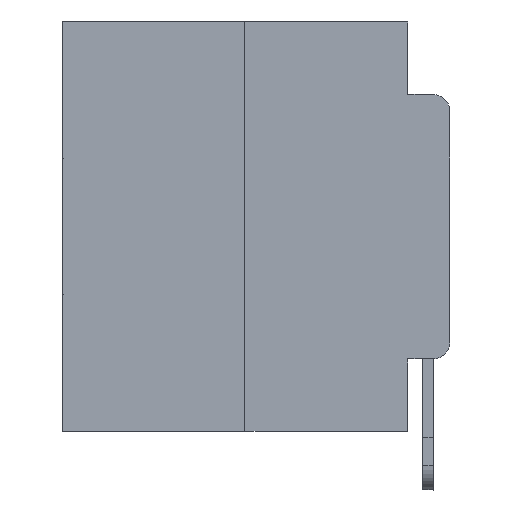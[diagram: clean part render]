
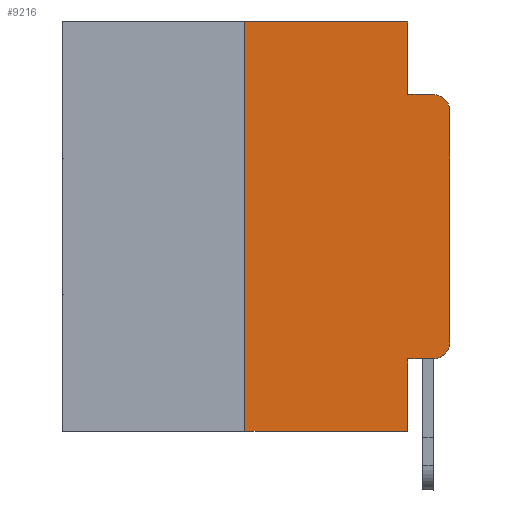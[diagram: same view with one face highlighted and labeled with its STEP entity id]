
A CAD part, left-side view. The second image highlights one B-rep face of the part: STEP entity #9216.
In plain terms, the highlighted planar face has unit normal (-1, 0, 0).
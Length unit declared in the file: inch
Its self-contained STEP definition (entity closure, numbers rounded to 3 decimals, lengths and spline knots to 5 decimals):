
#13 = ORIENTED_EDGE ( 'NONE', *, *, #11426, .T. ) ;
#339 = EDGE_LOOP ( 'NONE', ( #2021, #12326, #22945, #14389, #1131, #7064, #25097, #4851, #19824, #13 ) ) ;
#681 = LINE ( 'NONE', #26886, #8783 ) ;
#1131 = ORIENTED_EDGE ( 'NONE', *, *, #4697, .F. ) ;
#1873 = CARTESIAN_POINT ( 'NONE',  ( 0., 0.25, 0. ) ) ;
#2021 = ORIENTED_EDGE ( 'NONE', *, *, #10709, .T. ) ;
#2022 = CARTESIAN_POINT ( 'NONE',  ( 0., 0., -0.1085 ) ) ;
#2228 = LINE ( 'NONE', #4345, #5234 ) ;
#2272 = EDGE_CURVE ( 'NONE', #8594, #25533, #11271, .T. ) ;
#2673 = LINE ( 'NONE', #8734, #18664 ) ;
#3498 = VERTEX_POINT ( 'NONE', #1873 ) ;
#3677 = DIRECTION ( 'NONE',  ( 0., 0., -1. ) ) ;
#3854 = VERTEX_POINT ( 'NONE', #20963 ) ;
#4334 = DIRECTION ( 'NONE',  ( 0., -1., 0. ) ) ;
#4345 = CARTESIAN_POINT ( 'NONE',  ( 0., 0.051, 0. ) ) ;
#4522 = CARTESIAN_POINT ( 'NONE',  ( 0., 0.02, -0.1085 ) ) ;
#4670 = DIRECTION ( 'NONE',  ( 0., 0., -1. ) ) ;
#4697 = EDGE_CURVE ( 'NONE', #3498, #24384, #17443, .T. ) ;
#4851 = ORIENTED_EDGE ( 'NONE', *, *, #14386, .F. ) ;
#5234 = VECTOR ( 'NONE', #18848, 39.37008 ) ;
#5288 = VECTOR ( 'NONE', #15645, 39.37008 ) ;
#5634 = PLANE ( 'NONE',  #9244 ) ;
#5676 = DIRECTION ( 'NONE',  ( -1., 0., 0. ) ) ;
#5908 = DIRECTION ( 'NONE',  ( 0., 0., 1. ) ) ;
#6292 = AXIS2_PLACEMENT_3D ( 'NONE', #4522, #25795, #4670 ) ;
#7058 = CARTESIAN_POINT ( 'NONE',  ( 0., 0.473, -0.5 ) ) ;
#7064 = ORIENTED_EDGE ( 'NONE', *, *, #27646, .F. ) ;
#7193 = CARTESIAN_POINT ( 'NONE',  ( 0., 0.473, 0. ) ) ;
#7738 = EDGE_CURVE ( 'NONE', #24384, #8024, #2228, .T. ) ;
#7787 = CARTESIAN_POINT ( 'NONE',  ( 0., 0.02, -0.3915 ) ) ;
#7888 = AXIS2_PLACEMENT_3D ( 'NONE', #7787, #5676, #14278 ) ;
#8024 = VERTEX_POINT ( 'NONE', #12317 ) ;
#8447 = LINE ( 'NONE', #17051, #10581 ) ;
#8594 = VERTEX_POINT ( 'NONE', #2022 ) ;
#8734 = CARTESIAN_POINT ( 'NONE',  ( 0., 0.25, 0. ) ) ;
#8783 = VECTOR ( 'NONE', #22518, 39.37008 ) ;
#9216 = ADVANCED_FACE ( 'NONE', ( #16068 ), #5634, .F. ) ;
#9244 = AXIS2_PLACEMENT_3D ( 'NONE', #7193, #9324, #14233 ) ;
#9324 = DIRECTION ( 'NONE',  ( 1., 0., 0. ) ) ;
#10442 = CARTESIAN_POINT ( 'NONE',  ( 0., 0.051, 0. ) ) ;
#10581 = VECTOR ( 'NONE', #5908, 39.37008 ) ;
#10709 = EDGE_CURVE ( 'NONE', #12063, #8594, #8447, .T. ) ;
#10959 = EDGE_CURVE ( 'NONE', #18829, #21122, #681, .T. ) ;
#11271 = CIRCLE ( 'NONE', #6292, 0.02 ) ;
#11426 = EDGE_CURVE ( 'NONE', #21122, #12063, #20038, .T. ) ;
#12063 = VERTEX_POINT ( 'NONE', #24229 ) ;
#12317 = CARTESIAN_POINT ( 'NONE',  ( 0., 0.051, -0.0885 ) ) ;
#12326 = ORIENTED_EDGE ( 'NONE', *, *, #2272, .T. ) ;
#13111 = VECTOR ( 'NONE', #4334, 39.37008 ) ;
#13583 = CARTESIAN_POINT ( 'NONE',  ( 0., 0.02, -0.0885 ) ) ;
#13868 = CARTESIAN_POINT ( 'NONE',  ( 0., 0.25, -0.5 ) ) ;
#14233 = DIRECTION ( 'NONE',  ( 0., 0., -1. ) ) ;
#14278 = DIRECTION ( 'NONE',  ( 0., 0., -1. ) ) ;
#14386 = EDGE_CURVE ( 'NONE', #18829, #3854, #25514, .T. ) ;
#14389 = ORIENTED_EDGE ( 'NONE', *, *, #7738, .F. ) ;
#15645 = DIRECTION ( 'NONE',  ( 0., -1., 0. ) ) ;
#15809 = EDGE_CURVE ( 'NONE', #23366, #3854, #26366, .T. ) ;
#16068 = FACE_OUTER_BOUND ( 'NONE', #339, .T. ) ;
#17041 = LINE ( 'NONE', #18855, #24244 ) ;
#17051 = CARTESIAN_POINT ( 'NONE',  ( 0., 0., 0. ) ) ;
#17443 = LINE ( 'NONE', #26176, #13111 ) ;
#18664 = VECTOR ( 'NONE', #21697, 39.37008 ) ;
#18829 = VERTEX_POINT ( 'NONE', #26495 ) ;
#18848 = DIRECTION ( 'NONE',  ( 0., 0., -1. ) ) ;
#18855 = CARTESIAN_POINT ( 'NONE',  ( 0., 0.051, -0.0885 ) ) ;
#19824 = ORIENTED_EDGE ( 'NONE', *, *, #10959, .T. ) ;
#20038 = CIRCLE ( 'NONE', #7888, 0.02 ) ;
#20963 = CARTESIAN_POINT ( 'NONE',  ( 0., 0.051, -0.5 ) ) ;
#21017 = EDGE_CURVE ( 'NONE', #8024, #25533, #17041, .T. ) ;
#21122 = VERTEX_POINT ( 'NONE', #26336 ) ;
#21183 = CARTESIAN_POINT ( 'NONE',  ( 0., 0.051, 0. ) ) ;
#21697 = DIRECTION ( 'NONE',  ( 0., 0., 1. ) ) ;
#22518 = DIRECTION ( 'NONE',  ( 0., -1., 0. ) ) ;
#22945 = ORIENTED_EDGE ( 'NONE', *, *, #21017, .F. ) ;
#23366 = VERTEX_POINT ( 'NONE', #13868 ) ;
#24229 = CARTESIAN_POINT ( 'NONE',  ( 0., 0., -0.3915 ) ) ;
#24244 = VECTOR ( 'NONE', #27733, 39.37008 ) ;
#24384 = VERTEX_POINT ( 'NONE', #21183 ) ;
#25097 = ORIENTED_EDGE ( 'NONE', *, *, #15809, .T. ) ;
#25514 = LINE ( 'NONE', #10442, #25902 ) ;
#25533 = VERTEX_POINT ( 'NONE', #13583 ) ;
#25795 = DIRECTION ( 'NONE',  ( -1., 0., 0. ) ) ;
#25902 = VECTOR ( 'NONE', #3677, 39.37008 ) ;
#26176 = CARTESIAN_POINT ( 'NONE',  ( 0., 0.473, 0. ) ) ;
#26336 = CARTESIAN_POINT ( 'NONE',  ( 0., 0.02, -0.4115 ) ) ;
#26366 = LINE ( 'NONE', #7058, #5288 ) ;
#26495 = CARTESIAN_POINT ( 'NONE',  ( 0., 0.051, -0.4115 ) ) ;
#26886 = CARTESIAN_POINT ( 'NONE',  ( 0., 0.051, -0.4115 ) ) ;
#27646 = EDGE_CURVE ( 'NONE', #23366, #3498, #2673, .T. ) ;
#27733 = DIRECTION ( 'NONE',  ( 0., -1., 0. ) ) ;
